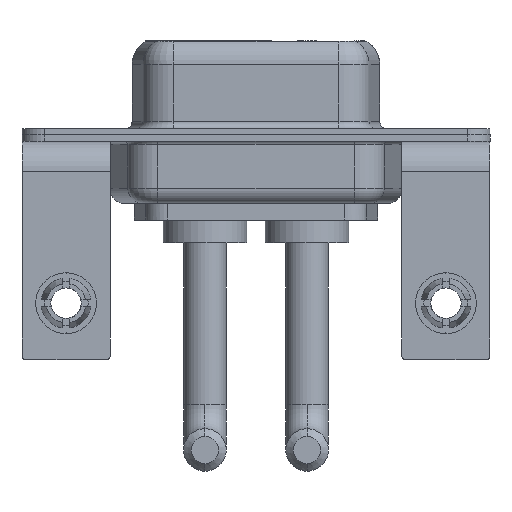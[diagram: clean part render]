
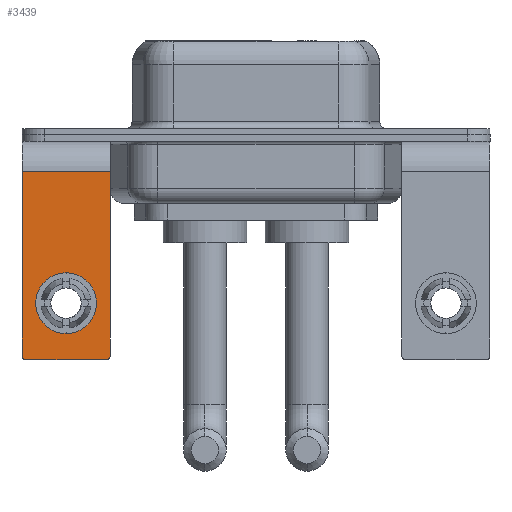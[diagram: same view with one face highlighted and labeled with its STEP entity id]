
A CAD part, front view. The second image highlights one B-rep face of the part: STEP entity #3439.
In plain terms, the highlighted planar face has unit normal (0, -1, 0).
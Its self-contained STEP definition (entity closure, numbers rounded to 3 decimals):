
#519 = VERTEX_POINT ( 'NONE', #14655 ) ;
#584 = CARTESIAN_POINT ( 'NONE',  ( 0., -6.25, -9.07 ) ) ;
#609 = LINE ( 'NONE', #842, #4468 ) ;
#842 = CARTESIAN_POINT ( 'NONE',  ( 2.9, -6.25, -14.8 ) ) ;
#851 = VERTEX_POINT ( 'NONE', #3657 ) ;
#997 = CARTESIAN_POINT ( 'NONE',  ( 2.9, -6.25, -2.4 ) ) ;
#1020 = CARTESIAN_POINT ( 'NONE',  ( 2.9, -6.25, -14.55 ) ) ;
#1202 = CIRCLE ( 'NONE', #14667, 0.25 ) ;
#1511 = ORIENTED_EDGE ( 'NONE', *, *, #8988, .T. ) ;
#1555 = FACE_OUTER_BOUND ( 'NONE', #12970, .T. ) ;
#1602 = EDGE_CURVE ( 'NONE', #4059, #12165, #1202, .T. ) ;
#1957 = DIRECTION ( 'NONE',  ( 0., 0., 1. ) ) ;
#2202 = EDGE_CURVE ( 'NONE', #14663, #7121, #10697, .T. ) ;
#2412 = DIRECTION ( 'NONE',  ( 0., 0., 1. ) ) ;
#2464 = ORIENTED_EDGE ( 'NONE', *, *, #8873, .T. ) ;
#2517 = DIRECTION ( 'NONE',  ( 0., 1., 0. ) ) ;
#2675 = AXIS2_PLACEMENT_3D ( 'NONE', #6727, #11580, #1957 ) ;
#2832 = AXIS2_PLACEMENT_3D ( 'NONE', #11260, #2517, #8633 ) ;
#3376 = DIRECTION ( 'NONE',  ( -1., 0., 0. ) ) ;
#3439 = ADVANCED_FACE ( 'NONE', ( #5002, #1555 ), #11018, .F. ) ;
#3657 = CARTESIAN_POINT ( 'NONE',  ( 2.65, -6.25, -14.8 ) ) ;
#3689 = AXIS2_PLACEMENT_3D ( 'NONE', #6566, #14978, #8939 ) ;
#4059 = VERTEX_POINT ( 'NONE', #6471 ) ;
#4138 = ORIENTED_EDGE ( 'NONE', *, *, #1602, .T. ) ;
#4447 = DIRECTION ( 'NONE',  ( 0., 0., 1. ) ) ;
#4468 = VECTOR ( 'NONE', #15157, 1000. ) ;
#4872 = AXIS2_PLACEMENT_3D ( 'NONE', #10689, #15531, #2412 ) ;
#5000 = CARTESIAN_POINT ( 'NONE',  ( -2.9, -6.25, -2.4 ) ) ;
#5002 = FACE_BOUND ( 'NONE', #8246, .T. ) ;
#5904 = ORIENTED_EDGE ( 'NONE', *, *, #14780, .T. ) ;
#5928 = CARTESIAN_POINT ( 'NONE',  ( 2.9, -6.25, -2.4 ) ) ;
#6471 = CARTESIAN_POINT ( 'NONE',  ( -2.9, -6.25, -14.55 ) ) ;
#6566 = CARTESIAN_POINT ( 'NONE',  ( 0., -6.25, -11.07 ) ) ;
#6727 = CARTESIAN_POINT ( 'NONE',  ( 2.65, -6.25, -14.55 ) ) ;
#7121 = VERTEX_POINT ( 'NONE', #1020 ) ;
#7137 = CIRCLE ( 'NONE', #4872, 2. ) ;
#7360 = DIRECTION ( 'NONE',  ( 0., 0., -1. ) ) ;
#8068 = EDGE_CURVE ( 'NONE', #11034, #519, #7137, .T. ) ;
#8087 = ORIENTED_EDGE ( 'NONE', *, *, #2202, .F. ) ;
#8246 = EDGE_LOOP ( 'NONE', ( #9751, #8734 ) ) ;
#8263 = VECTOR ( 'NONE', #3376, 1000. ) ;
#8633 = DIRECTION ( 'NONE',  ( 0., 0., 1. ) ) ;
#8734 = ORIENTED_EDGE ( 'NONE', *, *, #8068, .T. ) ;
#8810 = EDGE_CURVE ( 'NONE', #851, #12165, #609, .T. ) ;
#8873 = EDGE_CURVE ( 'NONE', #851, #7121, #13098, .T. ) ;
#8939 = DIRECTION ( 'NONE',  ( 0., 0., 1. ) ) ;
#8988 = EDGE_CURVE ( 'NONE', #12582, #4059, #14364, .T. ) ;
#9721 = LINE ( 'NONE', #5928, #8263 ) ;
#9751 = ORIENTED_EDGE ( 'NONE', *, *, #14527, .T. ) ;
#9933 = CARTESIAN_POINT ( 'NONE',  ( -2.65, -6.25, -14.8 ) ) ;
#10689 = CARTESIAN_POINT ( 'NONE',  ( 0., -6.25, -11.07 ) ) ;
#10697 = LINE ( 'NONE', #997, #13794 ) ;
#11018 = PLANE ( 'NONE',  #2832 ) ;
#11034 = VERTEX_POINT ( 'NONE', #584 ) ;
#11045 = CIRCLE ( 'NONE', #3689, 2. ) ;
#11260 = CARTESIAN_POINT ( 'NONE',  ( 2.9, -6.25, -2.4 ) ) ;
#11417 = CARTESIAN_POINT ( 'NONE',  ( -2.9, -6.25, -2.4 ) ) ;
#11580 = DIRECTION ( 'NONE',  ( 0., -1., 0. ) ) ;
#11748 = DIRECTION ( 'NONE',  ( 0., -1., 0. ) ) ;
#12165 = VERTEX_POINT ( 'NONE', #9933 ) ;
#12582 = VERTEX_POINT ( 'NONE', #11417 ) ;
#12970 = EDGE_LOOP ( 'NONE', ( #1511, #4138, #13014, #2464, #8087, #5904 ) ) ;
#13014 = ORIENTED_EDGE ( 'NONE', *, *, #8810, .F. ) ;
#13098 = CIRCLE ( 'NONE', #2675, 0.25 ) ;
#13794 = VECTOR ( 'NONE', #15544, 1000. ) ;
#14020 = CARTESIAN_POINT ( 'NONE',  ( 2.9, -6.25, -2.4 ) ) ;
#14144 = CARTESIAN_POINT ( 'NONE',  ( -2.65, -6.25, -14.55 ) ) ;
#14364 = LINE ( 'NONE', #5000, #14365 ) ;
#14365 = VECTOR ( 'NONE', #7360, 1000. ) ;
#14527 = EDGE_CURVE ( 'NONE', #519, #11034, #11045, .T. ) ;
#14655 = CARTESIAN_POINT ( 'NONE',  ( 0., -6.25, -13.07 ) ) ;
#14663 = VERTEX_POINT ( 'NONE', #14020 ) ;
#14667 = AXIS2_PLACEMENT_3D ( 'NONE', #14144, #11748, #4447 ) ;
#14780 = EDGE_CURVE ( 'NONE', #14663, #12582, #9721, .T. ) ;
#14978 = DIRECTION ( 'NONE',  ( 0., 1., 0. ) ) ;
#15157 = DIRECTION ( 'NONE',  ( -1., 0., 0. ) ) ;
#15531 = DIRECTION ( 'NONE',  ( 0., 1., 0. ) ) ;
#15544 = DIRECTION ( 'NONE',  ( 0., 0., -1. ) ) ;
